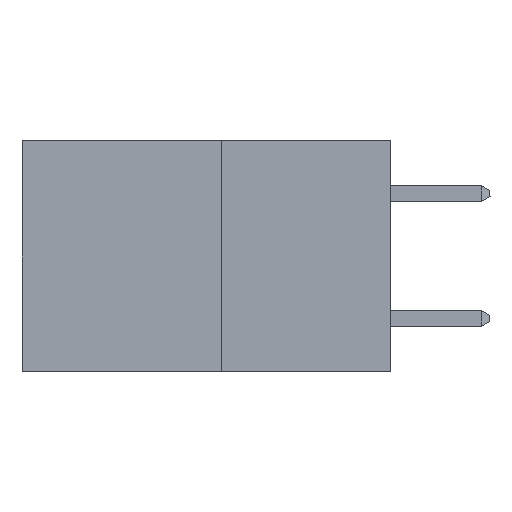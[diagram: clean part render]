
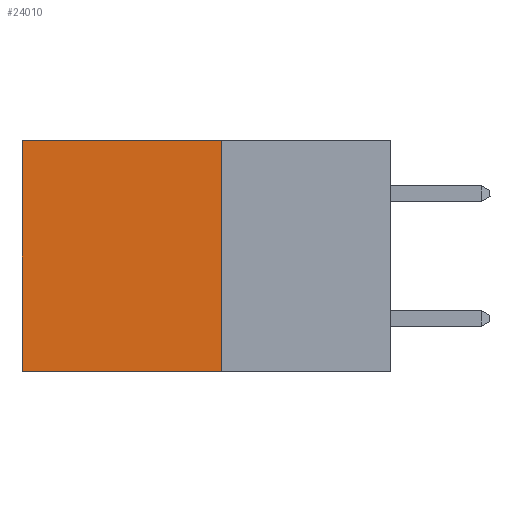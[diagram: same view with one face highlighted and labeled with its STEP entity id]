
A CAD part, left-side view. The second image highlights one B-rep face of the part: STEP entity #24010.
In plain terms, the highlighted planar face has unit normal (-1, 0, 0).
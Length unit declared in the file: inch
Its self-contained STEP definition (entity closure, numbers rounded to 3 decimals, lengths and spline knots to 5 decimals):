
#793 = CARTESIAN_POINT ( 'NONE',  ( 0.277, 0.59, -0.37 ) ) ;
#1118 = LINE ( 'NONE', #17108, #22349 ) ;
#1415 = CARTESIAN_POINT ( 'NONE',  ( 0.277, 0.27, -0.37 ) ) ;
#1615 = DIRECTION ( 'NONE',  ( 0., 1., 0. ) ) ;
#2219 = FACE_OUTER_BOUND ( 'NONE', #24984, .T. ) ;
#3513 = DIRECTION ( 'NONE',  ( 0., 0., -1. ) ) ;
#4373 = VERTEX_POINT ( 'NONE', #29850 ) ;
#4406 = LINE ( 'NONE', #33349, #17737 ) ;
#4833 = LINE ( 'NONE', #793, #18172 ) ;
#5188 = CARTESIAN_POINT ( 'NONE',  ( 0.277, 0.27, -0.37 ) ) ;
#6568 = VERTEX_POINT ( 'NONE', #16696 ) ;
#10349 = LINE ( 'NONE', #5188, #24390 ) ;
#11965 = CARTESIAN_POINT ( 'NONE',  ( 0.277, 0.59, -0.37 ) ) ;
#12025 = DIRECTION ( 'NONE',  ( 1., 0., 0. ) ) ;
#14585 = PLANE ( 'NONE',  #25692 ) ;
#15826 = ORIENTED_EDGE ( 'NONE', *, *, #28598, .T. ) ;
#16642 = EDGE_CURVE ( 'NONE', #4373, #28145, #10349, .T. ) ;
#16696 = CARTESIAN_POINT ( 'NONE',  ( 0.277, 0.59, 0. ) ) ;
#17108 = CARTESIAN_POINT ( 'NONE',  ( 0.277, 0.27, -0.37 ) ) ;
#17627 = EDGE_CURVE ( 'NONE', #28145, #25242, #1118, .T. ) ;
#17737 = VECTOR ( 'NONE', #1615, 39.37008 ) ;
#18172 = VECTOR ( 'NONE', #3513, 39.37008 ) ;
#18440 = ORIENTED_EDGE ( 'NONE', *, *, #28809, .T. ) ;
#22349 = VECTOR ( 'NONE', #32834, 39.37008 ) ;
#23707 = DIRECTION ( 'NONE',  ( 0., 0., -1. ) ) ;
#23931 = ORIENTED_EDGE ( 'NONE', *, *, #16642, .F. ) ;
#24010 = ADVANCED_FACE ( 'NONE', ( #2219 ), #14585, .F. ) ;
#24390 = VECTOR ( 'NONE', #23707, 39.37008 ) ;
#24984 = EDGE_LOOP ( 'NONE', ( #15826, #27376, #23931, #18440 ) ) ;
#25242 = VERTEX_POINT ( 'NONE', #11965 ) ;
#25692 = AXIS2_PLACEMENT_3D ( 'NONE', #27806, #12025, #30453 ) ;
#27376 = ORIENTED_EDGE ( 'NONE', *, *, #17627, .F. ) ;
#27806 = CARTESIAN_POINT ( 'NONE',  ( 0.277, 0.27, -0.37 ) ) ;
#28145 = VERTEX_POINT ( 'NONE', #1415 ) ;
#28598 = EDGE_CURVE ( 'NONE', #6568, #25242, #4833, .T. ) ;
#28809 = EDGE_CURVE ( 'NONE', #4373, #6568, #4406, .T. ) ;
#29850 = CARTESIAN_POINT ( 'NONE',  ( 0.277, 0.27, 0. ) ) ;
#30453 = DIRECTION ( 'NONE',  ( 0., 0., -1. ) ) ;
#32834 = DIRECTION ( 'NONE',  ( 0., 1., 0. ) ) ;
#33349 = CARTESIAN_POINT ( 'NONE',  ( 0.277, 0.27, 0. ) ) ;
